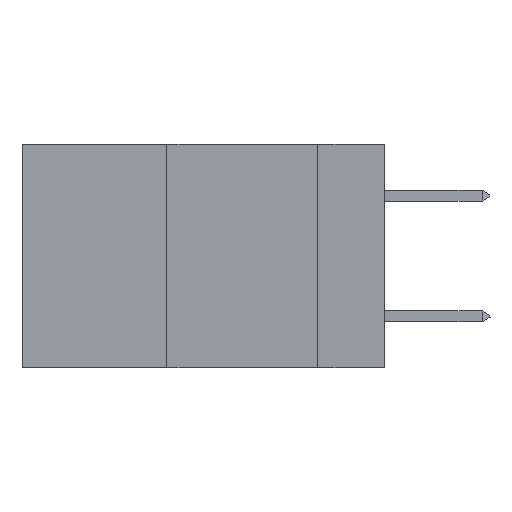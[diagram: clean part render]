
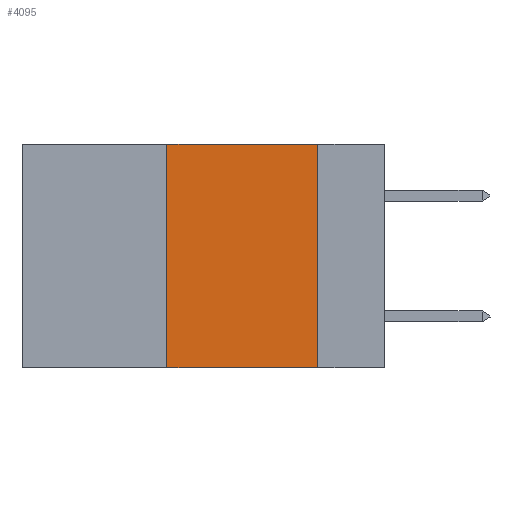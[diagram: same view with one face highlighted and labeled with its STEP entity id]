
A CAD part, left-side view. The second image highlights one B-rep face of the part: STEP entity #4095.
In plain terms, the highlighted planar face has unit normal (-1, 0, 0).
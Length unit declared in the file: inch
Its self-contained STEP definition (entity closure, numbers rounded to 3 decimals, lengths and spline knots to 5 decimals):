
#395 = DIRECTION ( 'NONE',  ( 1., 0., 0. ) ) ;
#1400 = DIRECTION ( 'NONE',  ( 0., 0., -1. ) ) ;
#2869 = LINE ( 'NONE', #26633, #14356 ) ;
#4095 = ADVANCED_FACE ( 'NONE', ( #7084 ), #20451, .F. ) ;
#4165 = VERTEX_POINT ( 'NONE', #31008 ) ;
#4917 = DIRECTION ( 'NONE',  ( 0., 0., 1. ) ) ;
#5114 = VERTEX_POINT ( 'NONE', #9523 ) ;
#5337 = ORIENTED_EDGE ( 'NONE', *, *, #19047, .F. ) ;
#5407 = CARTESIAN_POINT ( 'NONE',  ( 0., 0.6, 0. ) ) ;
#7084 = FACE_OUTER_BOUND ( 'NONE', #29844, .T. ) ;
#9348 = DIRECTION ( 'NONE',  ( 0., -1., 0. ) ) ;
#9523 = CARTESIAN_POINT ( 'NONE',  ( 0., 0.36, -0.37 ) ) ;
#14281 = ORIENTED_EDGE ( 'NONE', *, *, #18037, .T. ) ;
#14356 = VECTOR ( 'NONE', #1400, 39.37008 ) ;
#14550 = CARTESIAN_POINT ( 'NONE',  ( 0., 0.6, 0. ) ) ;
#14697 = LINE ( 'NONE', #26750, #16287 ) ;
#15583 = EDGE_CURVE ( 'NONE', #4165, #30542, #16880, .T. ) ;
#16287 = VECTOR ( 'NONE', #21732, 39.37008 ) ;
#16880 = LINE ( 'NONE', #14550, #21574 ) ;
#17982 = EDGE_CURVE ( 'NONE', #30542, #19667, #2869, .T. ) ;
#18037 = EDGE_CURVE ( 'NONE', #5114, #19667, #14697, .T. ) ;
#18385 = ORIENTED_EDGE ( 'NONE', *, *, #17982, .F. ) ;
#19047 = EDGE_CURVE ( 'NONE', #5114, #4165, #32057, .T. ) ;
#19667 = VERTEX_POINT ( 'NONE', #32380 ) ;
#20451 = PLANE ( 'NONE',  #28016 ) ;
#21574 = VECTOR ( 'NONE', #9348, 39.37008 ) ;
#21732 = DIRECTION ( 'NONE',  ( 0., -1., 0. ) ) ;
#22691 = DIRECTION ( 'NONE',  ( 0., 0., -1. ) ) ;
#25963 = VECTOR ( 'NONE', #4917, 39.37008 ) ;
#26633 = CARTESIAN_POINT ( 'NONE',  ( 0., 0.11, 0. ) ) ;
#26750 = CARTESIAN_POINT ( 'NONE',  ( 0., 0.6, -0.37 ) ) ;
#28016 = AXIS2_PLACEMENT_3D ( 'NONE', #5407, #395, #22691 ) ;
#29844 = EDGE_LOOP ( 'NONE', ( #18385, #30649, #5337, #14281 ) ) ;
#29912 = CARTESIAN_POINT ( 'NONE',  ( 0., 0.11, 0. ) ) ;
#30402 = CARTESIAN_POINT ( 'NONE',  ( 0., 0.36, 0. ) ) ;
#30542 = VERTEX_POINT ( 'NONE', #29912 ) ;
#30649 = ORIENTED_EDGE ( 'NONE', *, *, #15583, .F. ) ;
#31008 = CARTESIAN_POINT ( 'NONE',  ( 0., 0.36, 0. ) ) ;
#32057 = LINE ( 'NONE', #30402, #25963 ) ;
#32380 = CARTESIAN_POINT ( 'NONE',  ( 0., 0.11, -0.37 ) ) ;
